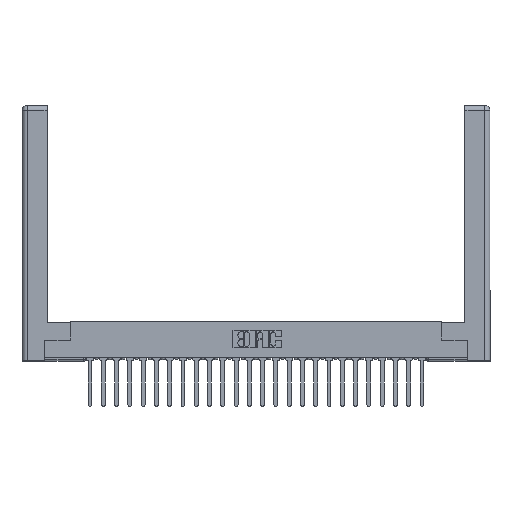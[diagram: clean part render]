
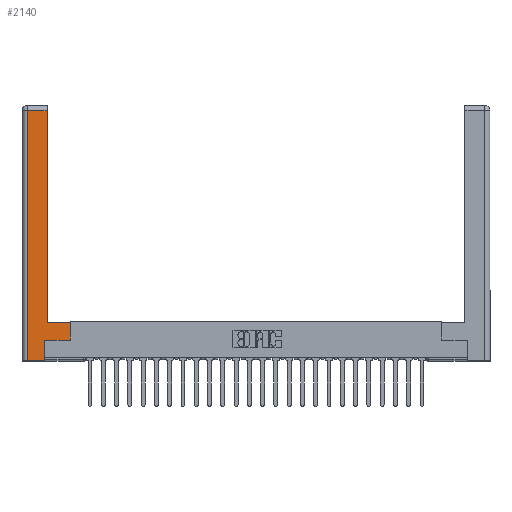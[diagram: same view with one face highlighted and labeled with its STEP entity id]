
A CAD part, top view. The second image highlights one B-rep face of the part: STEP entity #2140.
In plain terms, the highlighted planar face has unit normal (0, 0, 1).
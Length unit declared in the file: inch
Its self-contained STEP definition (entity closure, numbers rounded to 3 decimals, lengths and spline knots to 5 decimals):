
#393 = CARTESIAN_POINT ( 'NONE',  ( 0.295, 0.45, 0. ) ) ;
#641 = ORIENTED_EDGE ( 'NONE', *, *, #21835, .T. ) ;
#920 = CARTESIAN_POINT ( 'NONE',  ( 0.0615, 2.94, 0. ) ) ;
#935 = CARTESIAN_POINT ( 'NONE',  ( 0., 0., 0. ) ) ;
#1805 = CARTESIAN_POINT ( 'NONE',  ( 0.565, 0.45, 0. ) ) ;
#2140 = ADVANCED_FACE ( 'NONE', ( #13594 ), #23654, .F. ) ;
#3806 = LINE ( 'NONE', #9801, #20487 ) ;
#4023 = VECTOR ( 'NONE', #8967, 39.37008 ) ;
#4613 = CARTESIAN_POINT ( 'NONE',  ( 0.265, 0.245, 0. ) ) ;
#4832 = DIRECTION ( 'NONE',  ( -1., 0., 0. ) ) ;
#5262 = CARTESIAN_POINT ( 'NONE',  ( 0.295, 3., 0. ) ) ;
#5711 = VECTOR ( 'NONE', #10738, 39.37008 ) ;
#5922 = ORIENTED_EDGE ( 'NONE', *, *, #25472, .T. ) ;
#6480 = EDGE_CURVE ( 'NONE', #25049, #17726, #23363, .T. ) ;
#7316 = LINE ( 'NONE', #5262, #17980 ) ;
#7692 = EDGE_CURVE ( 'NONE', #8612, #23264, #19021, .T. ) ;
#8612 = VERTEX_POINT ( 'NONE', #1805 ) ;
#8643 = ORIENTED_EDGE ( 'NONE', *, *, #20250, .T. ) ;
#8967 = DIRECTION ( 'NONE',  ( -1., 0., 0. ) ) ;
#9076 = AXIS2_PLACEMENT_3D ( 'NONE', #935, #21488, #21884 ) ;
#9801 = CARTESIAN_POINT ( 'NONE',  ( 0.565, 0.45, 0. ) ) ;
#10133 = CARTESIAN_POINT ( 'NONE',  ( 0.0615, 0., 0. ) ) ;
#10273 = CARTESIAN_POINT ( 'NONE',  ( 0.295, 2.94, 0. ) ) ;
#10738 = DIRECTION ( 'NONE',  ( 1., 0., 0. ) ) ;
#11358 = ORIENTED_EDGE ( 'NONE', *, *, #12352, .T. ) ;
#11619 = CARTESIAN_POINT ( 'NONE',  ( 0.265, 0., 0. ) ) ;
#11847 = VECTOR ( 'NONE', #25423, 39.37008 ) ;
#12074 = CARTESIAN_POINT ( 'NONE',  ( 0.0615, 0., 0. ) ) ;
#12168 = VECTOR ( 'NONE', #25858, 39.37008 ) ;
#12249 = VERTEX_POINT ( 'NONE', #920 ) ;
#12352 = EDGE_CURVE ( 'NONE', #23264, #18374, #7316, .T. ) ;
#13465 = ORIENTED_EDGE ( 'NONE', *, *, #21756, .T. ) ;
#13574 = DIRECTION ( 'NONE',  ( 0., 1., 0. ) ) ;
#13594 = FACE_OUTER_BOUND ( 'NONE', #13747, .T. ) ;
#13747 = EDGE_LOOP ( 'NONE', ( #11358, #17541, #5922, #8643, #14008, #641, #13465, #26417 ) ) ;
#14008 = ORIENTED_EDGE ( 'NONE', *, *, #6480, .T. ) ;
#14503 = EDGE_CURVE ( 'NONE', #18374, #12249, #17754, .T. ) ;
#14775 = VECTOR ( 'NONE', #4832, 39.37008 ) ;
#15628 = CARTESIAN_POINT ( 'NONE',  ( 0.265, 0.245, 0. ) ) ;
#15954 = VERTEX_POINT ( 'NONE', #10133 ) ;
#17541 = ORIENTED_EDGE ( 'NONE', *, *, #14503, .T. ) ;
#17726 = VERTEX_POINT ( 'NONE', #15628 ) ;
#17754 = LINE ( 'NONE', #21568, #14775 ) ;
#17980 = VECTOR ( 'NONE', #13574, 39.37008 ) ;
#18374 = VERTEX_POINT ( 'NONE', #10273 ) ;
#18475 = LINE ( 'NONE', #12074, #20484 ) ;
#18567 = CARTESIAN_POINT ( 'NONE',  ( 0.565, 0.245, 0. ) ) ;
#19021 = LINE ( 'NONE', #393, #4023 ) ;
#19025 = LINE ( 'NONE', #22837, #5711 ) ;
#19431 = CARTESIAN_POINT ( 'NONE',  ( 0.295, 0.45, 0. ) ) ;
#20250 = EDGE_CURVE ( 'NONE', #15954, #25049, #25722, .T. ) ;
#20379 = DIRECTION ( 'NONE',  ( 0., 1., 0. ) ) ;
#20484 = VECTOR ( 'NONE', #22137, 39.37008 ) ;
#20487 = VECTOR ( 'NONE', #20379, 39.37008 ) ;
#21488 = DIRECTION ( 'NONE',  ( 0., 0., -1. ) ) ;
#21568 = CARTESIAN_POINT ( 'NONE',  ( 0.0615, 2.94, 0. ) ) ;
#21756 = EDGE_CURVE ( 'NONE', #24801, #8612, #3806, .T. ) ;
#21835 = EDGE_CURVE ( 'NONE', #17726, #24801, #19025, .T. ) ;
#21884 = DIRECTION ( 'NONE',  ( -1., 0., 0. ) ) ;
#22137 = DIRECTION ( 'NONE',  ( 0., -1., 0. ) ) ;
#22837 = CARTESIAN_POINT ( 'NONE',  ( 0.565, 0.245, 0. ) ) ;
#23264 = VERTEX_POINT ( 'NONE', #19431 ) ;
#23363 = LINE ( 'NONE', #4613, #11847 ) ;
#23654 = PLANE ( 'NONE',  #9076 ) ;
#24801 = VERTEX_POINT ( 'NONE', #18567 ) ;
#25049 = VERTEX_POINT ( 'NONE', #11619 ) ;
#25423 = DIRECTION ( 'NONE',  ( 0., 1., 0. ) ) ;
#25472 = EDGE_CURVE ( 'NONE', #12249, #15954, #18475, .T. ) ;
#25722 = LINE ( 'NONE', #26268, #12168 ) ;
#25858 = DIRECTION ( 'NONE',  ( 1., 0., 0. ) ) ;
#26268 = CARTESIAN_POINT ( 'NONE',  ( 0.265, 0., 0. ) ) ;
#26417 = ORIENTED_EDGE ( 'NONE', *, *, #7692, .T. ) ;
